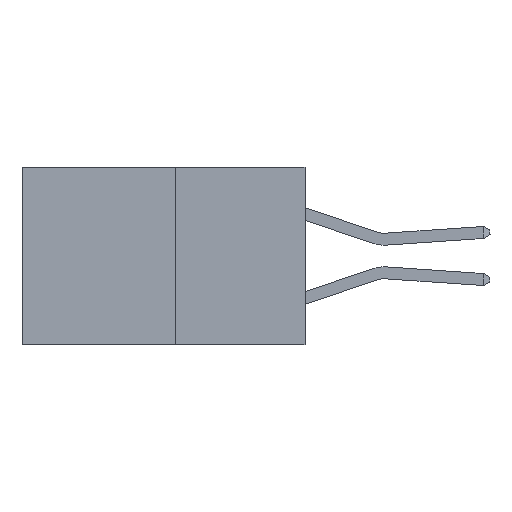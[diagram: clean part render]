
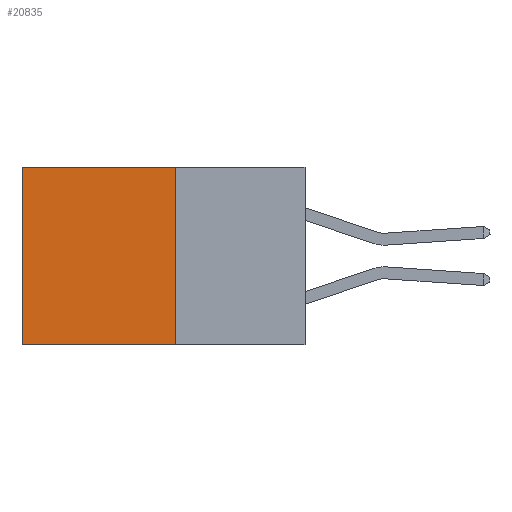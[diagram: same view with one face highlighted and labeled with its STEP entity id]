
A CAD part, left-side view. The second image highlights one B-rep face of the part: STEP entity #20835.
In plain terms, the highlighted planar face has unit normal (-1, 0, 0).
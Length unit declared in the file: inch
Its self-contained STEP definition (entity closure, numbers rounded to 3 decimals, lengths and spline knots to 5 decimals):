
#276 = CARTESIAN_POINT ( 'NONE',  ( 0.277, 0.59, -0.37 ) ) ;
#366 = CARTESIAN_POINT ( 'NONE',  ( 0.277, 0.27, 0. ) ) ;
#1922 = DIRECTION ( 'NONE',  ( 0., 0., -1. ) ) ;
#2081 = DIRECTION ( 'NONE',  ( 0., 1., 0. ) ) ;
#2204 = ORIENTED_EDGE ( 'NONE', *, *, #20922, .F. ) ;
#3964 = CARTESIAN_POINT ( 'NONE',  ( 0.277, 0.59, 0. ) ) ;
#5125 = EDGE_CURVE ( 'NONE', #11331, #14056, #14924, .T. ) ;
#5717 = ORIENTED_EDGE ( 'NONE', *, *, #5125, .T. ) ;
#5923 = ORIENTED_EDGE ( 'NONE', *, *, #19297, .F. ) ;
#6078 = CARTESIAN_POINT ( 'NONE',  ( 0.277, 0.27, -0.37 ) ) ;
#6303 = VECTOR ( 'NONE', #2081, 39.37008 ) ;
#7735 = FACE_OUTER_BOUND ( 'NONE', #22613, .T. ) ;
#8647 = CARTESIAN_POINT ( 'NONE',  ( 0.277, 0.27, 0. ) ) ;
#9783 = PLANE ( 'NONE',  #19321 ) ;
#11331 = VERTEX_POINT ( 'NONE', #366 ) ;
#11793 = CARTESIAN_POINT ( 'NONE',  ( 0.277, 0.27, -0.37 ) ) ;
#12080 = VECTOR ( 'NONE', #12693, 39.37008 ) ;
#12177 = EDGE_CURVE ( 'NONE', #14056, #21557, #17264, .T. ) ;
#12693 = DIRECTION ( 'NONE',  ( 0., 0., -1. ) ) ;
#13774 = DIRECTION ( 'NONE',  ( 1., 0., 0. ) ) ;
#14056 = VERTEX_POINT ( 'NONE', #3964 ) ;
#14924 = LINE ( 'NONE', #8647, #20086 ) ;
#15071 = DIRECTION ( 'NONE',  ( 0., 1., 0. ) ) ;
#15172 = LINE ( 'NONE', #6078, #19715 ) ;
#15751 = ORIENTED_EDGE ( 'NONE', *, *, #12177, .T. ) ;
#17264 = LINE ( 'NONE', #20445, #12080 ) ;
#17391 = LINE ( 'NONE', #23657, #6303 ) ;
#19297 = EDGE_CURVE ( 'NONE', #24008, #21557, #17391, .T. ) ;
#19321 = AXIS2_PLACEMENT_3D ( 'NONE', #11793, #13774, #1922 ) ;
#19715 = VECTOR ( 'NONE', #21796, 39.37008 ) ;
#20086 = VECTOR ( 'NONE', #15071, 39.37008 ) ;
#20445 = CARTESIAN_POINT ( 'NONE',  ( 0.277, 0.59, -0.37 ) ) ;
#20835 = ADVANCED_FACE ( 'NONE', ( #7735 ), #9783, .F. ) ;
#20922 = EDGE_CURVE ( 'NONE', #11331, #24008, #15172, .T. ) ;
#21557 = VERTEX_POINT ( 'NONE', #276 ) ;
#21796 = DIRECTION ( 'NONE',  ( 0., 0., -1. ) ) ;
#22613 = EDGE_LOOP ( 'NONE', ( #15751, #5923, #2204, #5717 ) ) ;
#23657 = CARTESIAN_POINT ( 'NONE',  ( 0.277, 0.27, -0.37 ) ) ;
#23864 = CARTESIAN_POINT ( 'NONE',  ( 0.277, 0.27, -0.37 ) ) ;
#24008 = VERTEX_POINT ( 'NONE', #23864 ) ;
